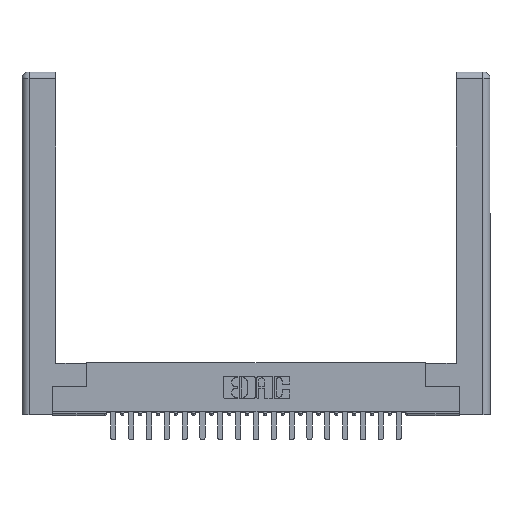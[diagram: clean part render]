
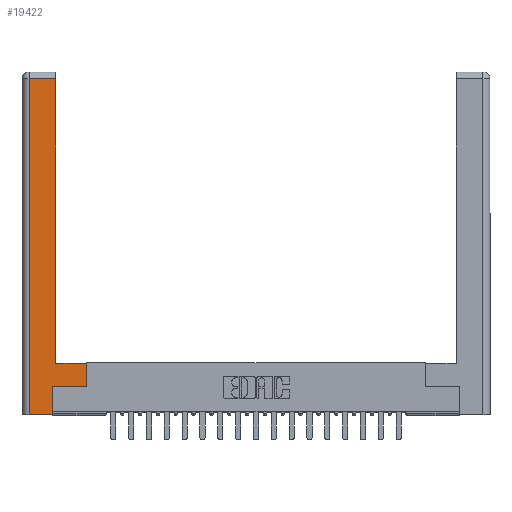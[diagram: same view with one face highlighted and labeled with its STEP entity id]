
A CAD part, top view. The second image highlights one B-rep face of the part: STEP entity #19422.
In plain terms, the highlighted planar face has unit normal (0, 0, 1).
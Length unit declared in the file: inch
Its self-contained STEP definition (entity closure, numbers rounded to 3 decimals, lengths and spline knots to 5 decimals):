
#100 = CARTESIAN_POINT ( 'NONE',  ( 0.295, 3., 0. ) ) ;
#820 = ORIENTED_EDGE ( 'NONE', *, *, #15984, .T. ) ;
#912 = CARTESIAN_POINT ( 'NONE',  ( 0.0615, 2.94, 0. ) ) ;
#1730 = VERTEX_POINT ( 'NONE', #17942 ) ;
#1780 = VERTEX_POINT ( 'NONE', #5163 ) ;
#2066 = DIRECTION ( 'NONE',  ( 0., -1., 0. ) ) ;
#2283 = CARTESIAN_POINT ( 'NONE',  ( 0.0615, 0., 0. ) ) ;
#2297 = EDGE_CURVE ( 'NONE', #19370, #1730, #4029, .T. ) ;
#2365 = DIRECTION ( 'NONE',  ( -1., 0., 0. ) ) ;
#2541 = ORIENTED_EDGE ( 'NONE', *, *, #9458, .T. ) ;
#2984 = VECTOR ( 'NONE', #18994, 39.37008 ) ;
#3005 = ORIENTED_EDGE ( 'NONE', *, *, #15447, .T. ) ;
#3102 = LINE ( 'NONE', #9879, #8799 ) ;
#3320 = EDGE_CURVE ( 'NONE', #5062, #1780, #6891, .T. ) ;
#3936 = VECTOR ( 'NONE', #20122, 39.37008 ) ;
#4029 = LINE ( 'NONE', #2283, #12570 ) ;
#4545 = EDGE_CURVE ( 'NONE', #1730, #11998, #3102, .T. ) ;
#5062 = VERTEX_POINT ( 'NONE', #10178 ) ;
#5163 = CARTESIAN_POINT ( 'NONE',  ( 0.565, 0.45, 0. ) ) ;
#5508 = VECTOR ( 'NONE', #16222, 39.37008 ) ;
#5618 = EDGE_LOOP ( 'NONE', ( #17449, #2541, #13672, #13511, #11350, #3005, #21527, #820 ) ) ;
#6350 = CARTESIAN_POINT ( 'NONE',  ( 0.295, 0.45, 0. ) ) ;
#6391 = VERTEX_POINT ( 'NONE', #19407 ) ;
#6891 = LINE ( 'NONE', #12291, #2984 ) ;
#7309 = CARTESIAN_POINT ( 'NONE',  ( 0.295, 2.94, 0. ) ) ;
#7372 = CARTESIAN_POINT ( 'NONE',  ( 0., 0., 0. ) ) ;
#7481 = FACE_OUTER_BOUND ( 'NONE', #5618, .T. ) ;
#8120 = VECTOR ( 'NONE', #17744, 39.37008 ) ;
#8226 = LINE ( 'NONE', #21513, #3936 ) ;
#8799 = VECTOR ( 'NONE', #9771, 39.37008 ) ;
#9458 = EDGE_CURVE ( 'NONE', #17839, #19370, #16109, .T. ) ;
#9771 = DIRECTION ( 'NONE',  ( 1., 0., 0. ) ) ;
#9873 = VERTEX_POINT ( 'NONE', #6350 ) ;
#9879 = CARTESIAN_POINT ( 'NONE',  ( 0.265, 0., 0. ) ) ;
#10178 = CARTESIAN_POINT ( 'NONE',  ( 0.565, 0.245, 0. ) ) ;
#10485 = DIRECTION ( 'NONE',  ( 0., 1., 0. ) ) ;
#10808 = CARTESIAN_POINT ( 'NONE',  ( 0.565, 0.245, 0. ) ) ;
#10811 = CARTESIAN_POINT ( 'NONE',  ( 0.265, 0.245, 0. ) ) ;
#11350 = ORIENTED_EDGE ( 'NONE', *, *, #16624, .T. ) ;
#11998 = VERTEX_POINT ( 'NONE', #14929 ) ;
#12291 = CARTESIAN_POINT ( 'NONE',  ( 0.565, 0.45, 0. ) ) ;
#12341 = VECTOR ( 'NONE', #10485, 39.37008 ) ;
#12570 = VECTOR ( 'NONE', #2066, 39.37008 ) ;
#12783 = VECTOR ( 'NONE', #21613, 39.37008 ) ;
#13500 = AXIS2_PLACEMENT_3D ( 'NONE', #7372, #17509, #2365 ) ;
#13511 = ORIENTED_EDGE ( 'NONE', *, *, #4545, .T. ) ;
#13672 = ORIENTED_EDGE ( 'NONE', *, *, #2297, .T. ) ;
#14671 = CARTESIAN_POINT ( 'NONE',  ( 0.0615, 2.94, 0. ) ) ;
#14929 = CARTESIAN_POINT ( 'NONE',  ( 0.265, 0., 0. ) ) ;
#15447 = EDGE_CURVE ( 'NONE', #6391, #5062, #17633, .T. ) ;
#15671 = LINE ( 'NONE', #10811, #12341 ) ;
#15984 = EDGE_CURVE ( 'NONE', #1780, #9873, #8226, .T. ) ;
#16109 = LINE ( 'NONE', #14671, #5508 ) ;
#16222 = DIRECTION ( 'NONE',  ( -1., 0., 0. ) ) ;
#16624 = EDGE_CURVE ( 'NONE', #11998, #6391, #15671, .T. ) ;
#17449 = ORIENTED_EDGE ( 'NONE', *, *, #19521, .T. ) ;
#17509 = DIRECTION ( 'NONE',  ( 0., 0., -1. ) ) ;
#17633 = LINE ( 'NONE', #10808, #8120 ) ;
#17744 = DIRECTION ( 'NONE',  ( 1., 0., 0. ) ) ;
#17839 = VERTEX_POINT ( 'NONE', #7309 ) ;
#17942 = CARTESIAN_POINT ( 'NONE',  ( 0.0615, 0., 0. ) ) ;
#18462 = LINE ( 'NONE', #100, #12783 ) ;
#18994 = DIRECTION ( 'NONE',  ( 0., 1., 0. ) ) ;
#19046 = PLANE ( 'NONE',  #13500 ) ;
#19370 = VERTEX_POINT ( 'NONE', #912 ) ;
#19407 = CARTESIAN_POINT ( 'NONE',  ( 0.265, 0.245, 0. ) ) ;
#19422 = ADVANCED_FACE ( 'NONE', ( #7481 ), #19046, .F. ) ;
#19521 = EDGE_CURVE ( 'NONE', #9873, #17839, #18462, .T. ) ;
#20122 = DIRECTION ( 'NONE',  ( -1., 0., 0. ) ) ;
#21513 = CARTESIAN_POINT ( 'NONE',  ( 0.295, 0.45, 0. ) ) ;
#21527 = ORIENTED_EDGE ( 'NONE', *, *, #3320, .T. ) ;
#21613 = DIRECTION ( 'NONE',  ( 0., 1., 0. ) ) ;
